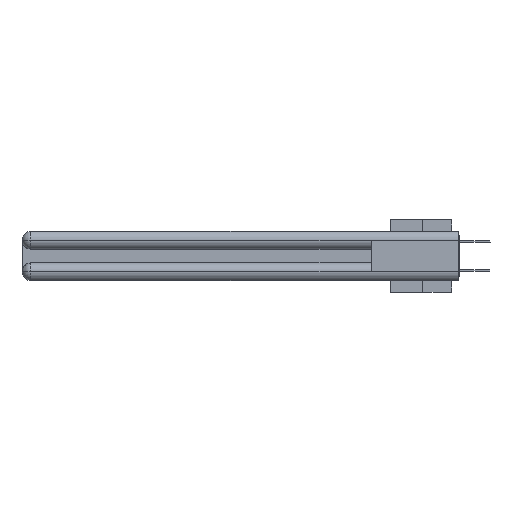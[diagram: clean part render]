
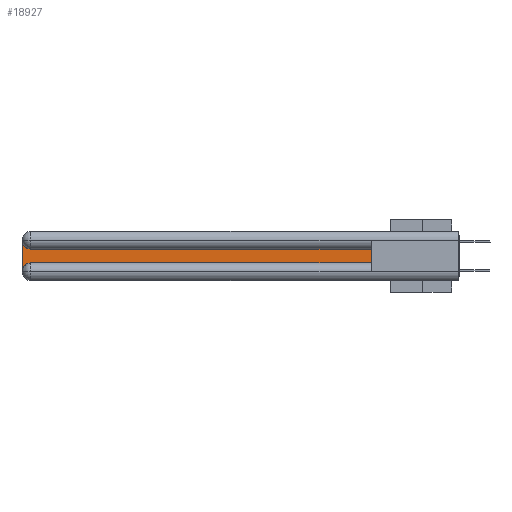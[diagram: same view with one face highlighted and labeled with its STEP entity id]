
A CAD part, left-side view. The second image highlights one B-rep face of the part: STEP entity #18927.
In plain terms, the highlighted planar face has unit normal (-1, 0, 0).
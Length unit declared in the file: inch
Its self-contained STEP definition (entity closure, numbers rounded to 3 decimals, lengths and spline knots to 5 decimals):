
#834 = CARTESIAN_POINT ( 'NONE',  ( 0.075, 0.6, -0.1225 ) ) ;
#2004 = ORIENTED_EDGE ( 'NONE', *, *, #2454, .T. ) ;
#2191 = ORIENTED_EDGE ( 'NONE', *, *, #15748, .T. ) ;
#2454 = EDGE_CURVE ( 'NONE', #13705, #13652, #33472, .T. ) ;
#3743 = LINE ( 'NONE', #834, #20577 ) ;
#6103 = DIRECTION ( 'NONE',  ( 1., 0., 0. ) ) ;
#6134 = VECTOR ( 'NONE', #21418, 39.37008 ) ;
#6397 = VECTOR ( 'NONE', #35033, 39.37008 ) ;
#7463 = CARTESIAN_POINT ( 'NONE',  ( 0.075, 2.94, -0.1225 ) ) ;
#7852 = CARTESIAN_POINT ( 'NONE',  ( 0.075, 3., -0.1225 ) ) ;
#12712 = AXIS2_PLACEMENT_3D ( 'NONE', #21097, #32966, #18566 ) ;
#12735 = VECTOR ( 'NONE', #25680, 39.37008 ) ;
#13652 = VERTEX_POINT ( 'NONE', #25223 ) ;
#13705 = VERTEX_POINT ( 'NONE', #34378 ) ;
#13771 = ORIENTED_EDGE ( 'NONE', *, *, #22046, .T. ) ;
#14906 = CARTESIAN_POINT ( 'NONE',  ( 0.075, 3., -0.0625 ) ) ;
#15247 = CARTESIAN_POINT ( 'NONE',  ( 0.075, 2.94, -0.2775 ) ) ;
#15748 = EDGE_CURVE ( 'NONE', #32038, #13705, #17904, .T. ) ;
#16141 = CARTESIAN_POINT ( 'NONE',  ( 0.075, 3., -0.2775 ) ) ;
#17904 = CIRCLE ( 'NONE', #31561, 0.06 ) ;
#18566 = DIRECTION ( 'NONE',  ( 0., 0., -1. ) ) ;
#18927 = ADVANCED_FACE ( 'NONE', ( #25765 ), #37048, .F. ) ;
#19081 = CARTESIAN_POINT ( 'NONE',  ( 0.075, 0.6, -0.2175 ) ) ;
#19163 = DIRECTION ( 'NONE',  ( 0., 0., -1. ) ) ;
#19930 = DIRECTION ( 'NONE',  ( 1., 0., 0. ) ) ;
#20577 = VECTOR ( 'NONE', #34084, 39.37008 ) ;
#21036 = CARTESIAN_POINT ( 'NONE',  ( 0.075, 0.6, -0.2175 ) ) ;
#21097 = CARTESIAN_POINT ( 'NONE',  ( 0.075, 2.94, -0.0625 ) ) ;
#21418 = DIRECTION ( 'NONE',  ( 0., -1., 0. ) ) ;
#22046 = EDGE_CURVE ( 'NONE', #30830, #32038, #25683, .T. ) ;
#22374 = LINE ( 'NONE', #19081, #12735 ) ;
#23158 = CARTESIAN_POINT ( 'NONE',  ( 0.075, 3., -0.2175 ) ) ;
#25223 = CARTESIAN_POINT ( 'NONE',  ( 0.075, 0.6, -0.2175 ) ) ;
#25680 = DIRECTION ( 'NONE',  ( 0., 0., 1. ) ) ;
#25683 = LINE ( 'NONE', #23158, #6397 ) ;
#25765 = FACE_OUTER_BOUND ( 'NONE', #31236, .T. ) ;
#26136 = CARTESIAN_POINT ( 'NONE',  ( 0.075, 0.6, -0.1225 ) ) ;
#27644 = VERTEX_POINT ( 'NONE', #26136 ) ;
#28027 = ORIENTED_EDGE ( 'NONE', *, *, #29067, .T. ) ;
#29067 = EDGE_CURVE ( 'NONE', #27644, #38053, #3743, .T. ) ;
#29845 = DIRECTION ( 'NONE',  ( 0., 0., -1. ) ) ;
#29901 = AXIS2_PLACEMENT_3D ( 'NONE', #7852, #19930, #19163 ) ;
#30830 = VERTEX_POINT ( 'NONE', #14906 ) ;
#31078 = ORIENTED_EDGE ( 'NONE', *, *, #33240, .T. ) ;
#31236 = EDGE_LOOP ( 'NONE', ( #28027, #32649, #13771, #2191, #2004, #31078 ) ) ;
#31561 = AXIS2_PLACEMENT_3D ( 'NONE', #15247, #6103, #29845 ) ;
#32038 = VERTEX_POINT ( 'NONE', #16141 ) ;
#32604 = CIRCLE ( 'NONE', #12712, 0.06 ) ;
#32649 = ORIENTED_EDGE ( 'NONE', *, *, #32675, .T. ) ;
#32675 = EDGE_CURVE ( 'NONE', #38053, #30830, #32604, .T. ) ;
#32966 = DIRECTION ( 'NONE',  ( 1., 0., 0. ) ) ;
#33240 = EDGE_CURVE ( 'NONE', #13652, #27644, #22374, .T. ) ;
#33472 = LINE ( 'NONE', #21036, #6134 ) ;
#34084 = DIRECTION ( 'NONE',  ( 0., 1., 0. ) ) ;
#34378 = CARTESIAN_POINT ( 'NONE',  ( 0.075, 2.94, -0.2175 ) ) ;
#35033 = DIRECTION ( 'NONE',  ( 0., 0., -1. ) ) ;
#37048 = PLANE ( 'NONE',  #29901 ) ;
#38053 = VERTEX_POINT ( 'NONE', #7463 ) ;
